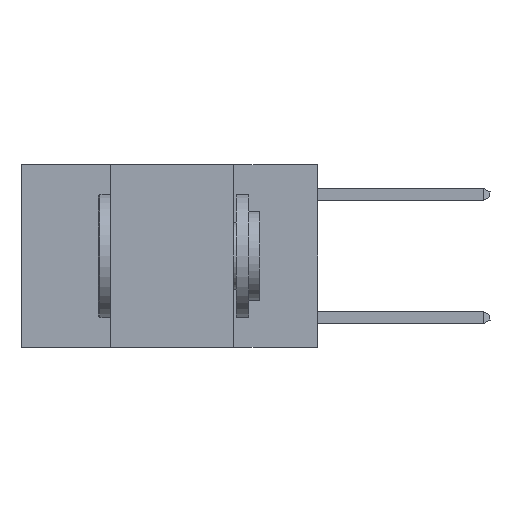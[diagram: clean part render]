
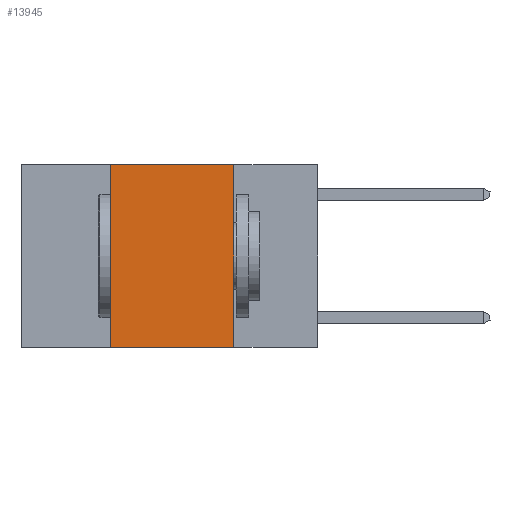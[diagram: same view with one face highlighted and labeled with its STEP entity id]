
A CAD part, left-side view. The second image highlights one B-rep face of the part: STEP entity #13945.
In plain terms, the highlighted planar face has unit normal (-1, 0, 0).
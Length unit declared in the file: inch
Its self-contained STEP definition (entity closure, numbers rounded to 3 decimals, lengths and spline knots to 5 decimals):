
#321 = PLANE ( 'NONE',  #20772 ) ;
#1065 = CARTESIAN_POINT ( 'NONE',  ( 0., 0.6, 0. ) ) ;
#1928 = DIRECTION ( 'NONE',  ( 0., 0., -1. ) ) ;
#4010 = CARTESIAN_POINT ( 'NONE',  ( 0., 0.17, -0.37 ) ) ;
#4056 = VECTOR ( 'NONE', #12311, 39.37008 ) ;
#4381 = DIRECTION ( 'NONE',  ( 0., 0., -1. ) ) ;
#4498 = CARTESIAN_POINT ( 'NONE',  ( 0., 0.17, 0. ) ) ;
#6072 = DIRECTION ( 'NONE',  ( 0., -1., 0. ) ) ;
#6215 = VERTEX_POINT ( 'NONE', #13044 ) ;
#7270 = CARTESIAN_POINT ( 'NONE',  ( 0., 0.6, 0. ) ) ;
#7810 = CARTESIAN_POINT ( 'NONE',  ( 0., 0.42, 0. ) ) ;
#8287 = ORIENTED_EDGE ( 'NONE', *, *, #22372, .F. ) ;
#8345 = ORIENTED_EDGE ( 'NONE', *, *, #21745, .F. ) ;
#9328 = CARTESIAN_POINT ( 'NONE',  ( 0., 0.17, 0. ) ) ;
#10617 = FACE_OUTER_BOUND ( 'NONE', #12745, .T. ) ;
#11135 = ORIENTED_EDGE ( 'NONE', *, *, #16674, .F. ) ;
#11706 = DIRECTION ( 'NONE',  ( 0., 0., 1. ) ) ;
#12177 = VERTEX_POINT ( 'NONE', #9328 ) ;
#12311 = DIRECTION ( 'NONE',  ( 0., -1., 0. ) ) ;
#12745 = EDGE_LOOP ( 'NONE', ( #8287, #8345, #11135, #19970 ) ) ;
#13044 = CARTESIAN_POINT ( 'NONE',  ( 0., 0.42, -0.37 ) ) ;
#13406 = VECTOR ( 'NONE', #6072, 39.37008 ) ;
#13903 = EDGE_CURVE ( 'NONE', #6215, #19096, #17618, .T. ) ;
#13945 = ADVANCED_FACE ( 'NONE', ( #10617 ), #321, .F. ) ;
#16327 = LINE ( 'NONE', #4498, #21341 ) ;
#16674 = EDGE_CURVE ( 'NONE', #6215, #20045, #18795, .T. ) ;
#17511 = DIRECTION ( 'NONE',  ( 1., 0., 0. ) ) ;
#17618 = LINE ( 'NONE', #20803, #4056 ) ;
#18247 = VECTOR ( 'NONE', #11706, 39.37008 ) ;
#18353 = LINE ( 'NONE', #1065, #13406 ) ;
#18795 = LINE ( 'NONE', #20284, #18247 ) ;
#19096 = VERTEX_POINT ( 'NONE', #4010 ) ;
#19970 = ORIENTED_EDGE ( 'NONE', *, *, #13903, .T. ) ;
#20045 = VERTEX_POINT ( 'NONE', #7810 ) ;
#20284 = CARTESIAN_POINT ( 'NONE',  ( 0., 0.42, 0. ) ) ;
#20772 = AXIS2_PLACEMENT_3D ( 'NONE', #7270, #17511, #1928 ) ;
#20803 = CARTESIAN_POINT ( 'NONE',  ( 0., 0.6, -0.37 ) ) ;
#21341 = VECTOR ( 'NONE', #4381, 39.37008 ) ;
#21745 = EDGE_CURVE ( 'NONE', #20045, #12177, #18353, .T. ) ;
#22372 = EDGE_CURVE ( 'NONE', #12177, #19096, #16327, .T. ) ;
